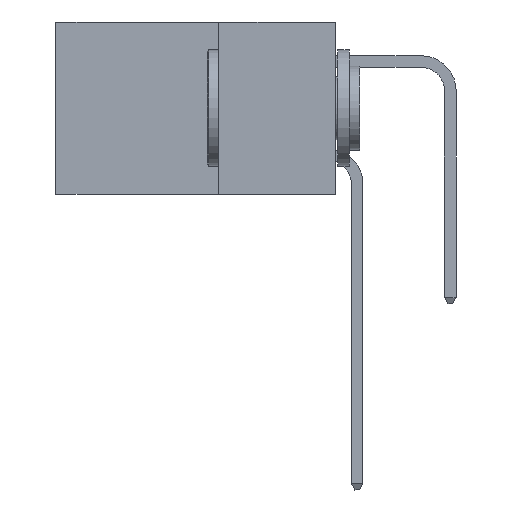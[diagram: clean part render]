
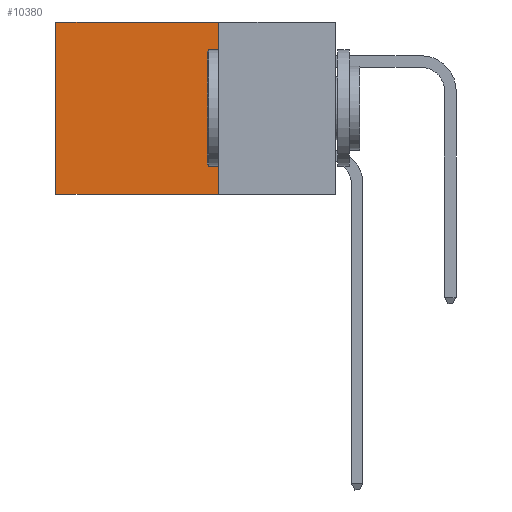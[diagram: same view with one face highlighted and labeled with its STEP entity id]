
A CAD part, left-side view. The second image highlights one B-rep face of the part: STEP entity #10380.
In plain terms, the highlighted planar face has unit normal (-1, 0, 0).
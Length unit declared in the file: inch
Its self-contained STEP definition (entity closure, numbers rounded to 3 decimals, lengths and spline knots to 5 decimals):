
#395 = VERTEX_POINT ( 'NONE', #4529 ) ;
#740 = AXIS2_PLACEMENT_3D ( 'NONE', #6242, #7233, #2555 ) ;
#1367 = ORIENTED_EDGE ( 'NONE', *, *, #7822, .F. ) ;
#1383 = FACE_OUTER_BOUND ( 'NONE', #5038, .T. ) ;
#1502 = ORIENTED_EDGE ( 'NONE', *, *, #2897, .T. ) ;
#2051 = DIRECTION ( 'NONE',  ( 0., 1., 0. ) ) ;
#2095 = VERTEX_POINT ( 'NONE', #5775 ) ;
#2555 = DIRECTION ( 'NONE',  ( 0., 0., -1. ) ) ;
#2897 = EDGE_CURVE ( 'NONE', #10199, #395, #3432, .T. ) ;
#3432 = LINE ( 'NONE', #9704, #11593 ) ;
#3902 = VERTEX_POINT ( 'NONE', #10107 ) ;
#4095 = DIRECTION ( 'NONE',  ( 0., 1., 0. ) ) ;
#4324 = VECTOR ( 'NONE', #9662, 39.37008 ) ;
#4529 = CARTESIAN_POINT ( 'NONE',  ( 0.2875, 0.6, -0.37 ) ) ;
#4625 = VECTOR ( 'NONE', #4095, 39.37008 ) ;
#4834 = CARTESIAN_POINT ( 'NONE',  ( 0.2875, 0.25, -0.37 ) ) ;
#5038 = EDGE_LOOP ( 'NONE', ( #1502, #5618, #1367, #8968 ) ) ;
#5192 = DIRECTION ( 'NONE',  ( 0., 0., -1. ) ) ;
#5618 = ORIENTED_EDGE ( 'NONE', *, *, #6466, .F. ) ;
#5775 = CARTESIAN_POINT ( 'NONE',  ( 0.2875, 0.25, 0. ) ) ;
#6242 = CARTESIAN_POINT ( 'NONE',  ( 0.2875, 0.25, 0. ) ) ;
#6466 = EDGE_CURVE ( 'NONE', #3902, #395, #10328, .T. ) ;
#6639 = EDGE_CURVE ( 'NONE', #2095, #10199, #10596, .T. ) ;
#7233 = DIRECTION ( 'NONE',  ( 1., 0., 0. ) ) ;
#7822 = EDGE_CURVE ( 'NONE', #2095, #3902, #9879, .T. ) ;
#7918 = VECTOR ( 'NONE', #2051, 39.37008 ) ;
#8893 = PLANE ( 'NONE',  #740 ) ;
#8968 = ORIENTED_EDGE ( 'NONE', *, *, #6639, .T. ) ;
#9434 = CARTESIAN_POINT ( 'NONE',  ( 0.2875, 0.25, 0. ) ) ;
#9546 = CARTESIAN_POINT ( 'NONE',  ( 0.2875, 0.25, 0. ) ) ;
#9662 = DIRECTION ( 'NONE',  ( 0., 0., -1. ) ) ;
#9704 = CARTESIAN_POINT ( 'NONE',  ( 0.2875, 0.6, 0. ) ) ;
#9879 = LINE ( 'NONE', #9546, #4324 ) ;
#9964 = CARTESIAN_POINT ( 'NONE',  ( 0.2875, 0.6, 0. ) ) ;
#10107 = CARTESIAN_POINT ( 'NONE',  ( 0.2875, 0.25, -0.37 ) ) ;
#10199 = VERTEX_POINT ( 'NONE', #9964 ) ;
#10328 = LINE ( 'NONE', #4834, #7918 ) ;
#10380 = ADVANCED_FACE ( 'NONE', ( #1383 ), #8893, .F. ) ;
#10596 = LINE ( 'NONE', #9434, #4625 ) ;
#11593 = VECTOR ( 'NONE', #5192, 39.37008 ) ;
